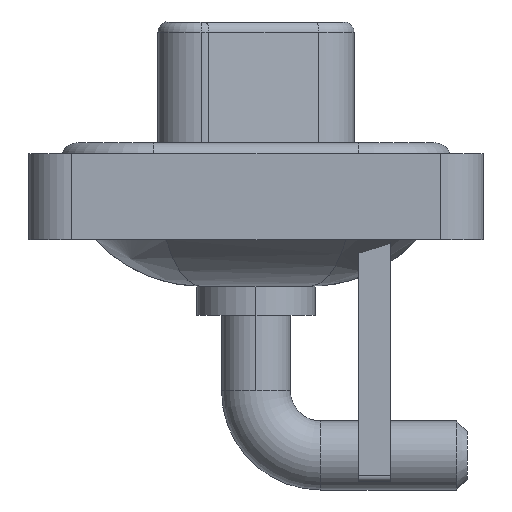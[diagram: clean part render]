
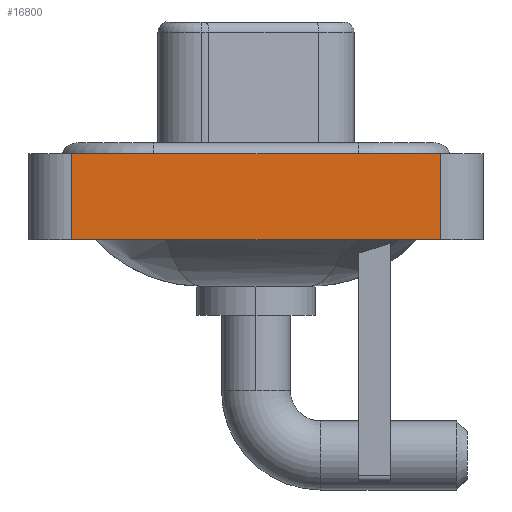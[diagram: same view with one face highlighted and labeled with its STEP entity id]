
A CAD part, left-side view. The second image highlights one B-rep face of the part: STEP entity #16800.
In plain terms, the highlighted planar face has unit normal (-1, 0, 0).
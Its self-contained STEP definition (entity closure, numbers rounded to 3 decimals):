
#161 = FACE_OUTER_BOUND ( 'NONE', #6757, .T. ) ;
#490 = DIRECTION ( 'NONE',  ( 0., -1., 0. ) ) ;
#985 = CARTESIAN_POINT ( 'NONE',  ( -7.3, -8.55, 0.4 ) ) ;
#1707 = CARTESIAN_POINT ( 'NONE',  ( -7.3, 8.55, -3.6 ) ) ;
#2275 = VECTOR ( 'NONE', #8822, 1000. ) ;
#2435 = DIRECTION ( 'NONE',  ( 0., 0., 1. ) ) ;
#2597 = CARTESIAN_POINT ( 'NONE',  ( -7.3, -8.55, -3.6 ) ) ;
#2710 = DIRECTION ( 'NONE',  ( 0., -1., 0. ) ) ;
#5356 = VERTEX_POINT ( 'NONE', #985 ) ;
#5688 = CARTESIAN_POINT ( 'NONE',  ( -7.3, -8.55, -3.6 ) ) ;
#5792 = EDGE_CURVE ( 'NONE', #12886, #5356, #9574, .T. ) ;
#6037 = CARTESIAN_POINT ( 'NONE',  ( -7.3, 8.55, 0.4 ) ) ;
#6607 = PLANE ( 'NONE',  #16174 ) ;
#6704 = VECTOR ( 'NONE', #16743, 1000. ) ;
#6757 = EDGE_LOOP ( 'NONE', ( #12146, #9817, #14321, #16623 ) ) ;
#8279 = CARTESIAN_POINT ( 'NONE',  ( -7.3, -8.55, -3.6 ) ) ;
#8822 = DIRECTION ( 'NONE',  ( 0., 0., 1. ) ) ;
#9574 = LINE ( 'NONE', #8279, #6704 ) ;
#9725 = EDGE_CURVE ( 'NONE', #16419, #12886, #11053, .T. ) ;
#9756 = VERTEX_POINT ( 'NONE', #6037 ) ;
#9817 = ORIENTED_EDGE ( 'NONE', *, *, #12504, .F. ) ;
#10149 = LINE ( 'NONE', #15485, #2275 ) ;
#11053 = LINE ( 'NONE', #5688, #12989 ) ;
#12146 = ORIENTED_EDGE ( 'NONE', *, *, #5792, .T. ) ;
#12163 = LINE ( 'NONE', #13727, #16209 ) ;
#12205 = EDGE_CURVE ( 'NONE', #16419, #9756, #10149, .T. ) ;
#12504 = EDGE_CURVE ( 'NONE', #9756, #5356, #12163, .T. ) ;
#12886 = VERTEX_POINT ( 'NONE', #13440 ) ;
#12989 = VECTOR ( 'NONE', #490, 1000. ) ;
#13440 = CARTESIAN_POINT ( 'NONE',  ( -7.3, -8.55, -3.6 ) ) ;
#13727 = CARTESIAN_POINT ( 'NONE',  ( -7.3, -8.55, 0.4 ) ) ;
#14321 = ORIENTED_EDGE ( 'NONE', *, *, #12205, .F. ) ;
#15485 = CARTESIAN_POINT ( 'NONE',  ( -7.3, 8.55, -3.6 ) ) ;
#15979 = DIRECTION ( 'NONE',  ( -1., 0., 0. ) ) ;
#16174 = AXIS2_PLACEMENT_3D ( 'NONE', #2597, #15979, #2435 ) ;
#16209 = VECTOR ( 'NONE', #2710, 1000. ) ;
#16419 = VERTEX_POINT ( 'NONE', #1707 ) ;
#16623 = ORIENTED_EDGE ( 'NONE', *, *, #9725, .T. ) ;
#16743 = DIRECTION ( 'NONE',  ( 0., 0., 1. ) ) ;
#16800 = ADVANCED_FACE ( 'NONE', ( #161 ), #6607, .T. ) ;
